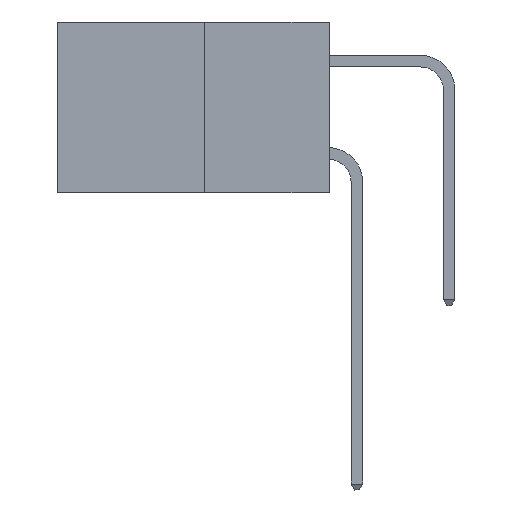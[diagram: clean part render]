
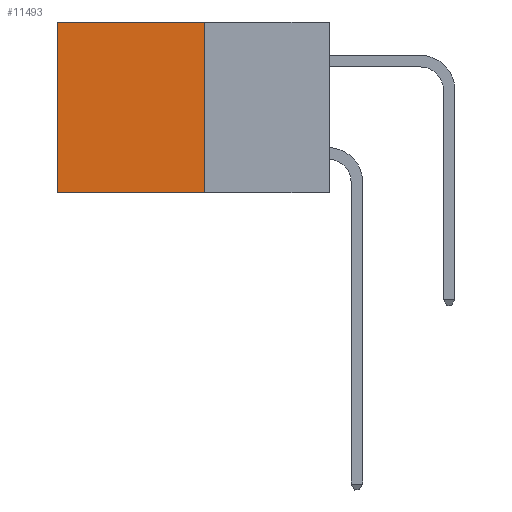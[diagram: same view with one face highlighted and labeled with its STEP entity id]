
A CAD part, left-side view. The second image highlights one B-rep face of the part: STEP entity #11493.
In plain terms, the highlighted planar face has unit normal (-1, 0, 0).
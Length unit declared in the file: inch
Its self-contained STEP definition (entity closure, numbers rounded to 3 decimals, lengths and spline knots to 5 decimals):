
#496 = LINE ( 'NONE', #32748, #7491 ) ;
#2396 = VERTEX_POINT ( 'NONE', #22383 ) ;
#4511 = ORIENTED_EDGE ( 'NONE', *, *, #29518, .T. ) ;
#4712 = DIRECTION ( 'NONE',  ( 0., 1., 0. ) ) ;
#6181 = DIRECTION ( 'NONE',  ( 1., 0., 0. ) ) ;
#6405 = DIRECTION ( 'NONE',  ( 0., 0., -1. ) ) ;
#7491 = VECTOR ( 'NONE', #6405, 39.37008 ) ;
#9605 = LINE ( 'NONE', #11476, #24333 ) ;
#11127 = FACE_OUTER_BOUND ( 'NONE', #27957, .T. ) ;
#11128 = EDGE_CURVE ( 'NONE', #20844, #2396, #496, .T. ) ;
#11476 = CARTESIAN_POINT ( 'NONE',  ( 0.277, 0.27, 0. ) ) ;
#11493 = ADVANCED_FACE ( 'NONE', ( #11127 ), #23788, .F. ) ;
#11888 = EDGE_CURVE ( 'NONE', #2396, #21124, #37280, .T. ) ;
#12100 = CARTESIAN_POINT ( 'NONE',  ( 0.277, 0.27, 0. ) ) ;
#12962 = VECTOR ( 'NONE', #4712, 39.37008 ) ;
#14312 = ORIENTED_EDGE ( 'NONE', *, *, #11128, .F. ) ;
#14441 = DIRECTION ( 'NONE',  ( 0., 1., 0. ) ) ;
#14901 = CARTESIAN_POINT ( 'NONE',  ( 0.277, 0.27, -0.37 ) ) ;
#16094 = DIRECTION ( 'NONE',  ( 0., 0., -1. ) ) ;
#18668 = LINE ( 'NONE', #22038, #25547 ) ;
#20844 = VERTEX_POINT ( 'NONE', #12100 ) ;
#21091 = VERTEX_POINT ( 'NONE', #24918 ) ;
#21124 = VERTEX_POINT ( 'NONE', #22103 ) ;
#22038 = CARTESIAN_POINT ( 'NONE',  ( 0.277, 0.59, -0.37 ) ) ;
#22103 = CARTESIAN_POINT ( 'NONE',  ( 0.277, 0.59, -0.37 ) ) ;
#22383 = CARTESIAN_POINT ( 'NONE',  ( 0.277, 0.27, -0.37 ) ) ;
#23788 = PLANE ( 'NONE',  #34373 ) ;
#24333 = VECTOR ( 'NONE', #14441, 39.37008 ) ;
#24918 = CARTESIAN_POINT ( 'NONE',  ( 0.277, 0.59, 0. ) ) ;
#25547 = VECTOR ( 'NONE', #16094, 39.37008 ) ;
#26706 = ORIENTED_EDGE ( 'NONE', *, *, #11888, .F. ) ;
#26736 = DIRECTION ( 'NONE',  ( 0., 0., -1. ) ) ;
#27957 = EDGE_LOOP ( 'NONE', ( #4511, #26706, #14312, #28749 ) ) ;
#28248 = CARTESIAN_POINT ( 'NONE',  ( 0.277, 0.27, -0.37 ) ) ;
#28749 = ORIENTED_EDGE ( 'NONE', *, *, #33459, .T. ) ;
#29518 = EDGE_CURVE ( 'NONE', #21091, #21124, #18668, .T. ) ;
#32748 = CARTESIAN_POINT ( 'NONE',  ( 0.277, 0.27, -0.37 ) ) ;
#33459 = EDGE_CURVE ( 'NONE', #20844, #21091, #9605, .T. ) ;
#34373 = AXIS2_PLACEMENT_3D ( 'NONE', #14901, #6181, #26736 ) ;
#37280 = LINE ( 'NONE', #28248, #12962 ) ;
